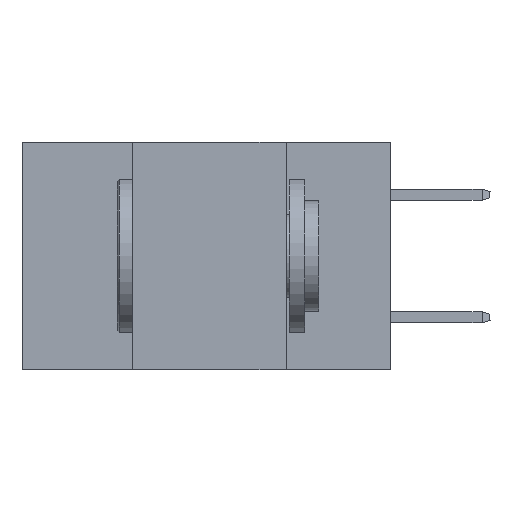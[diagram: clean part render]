
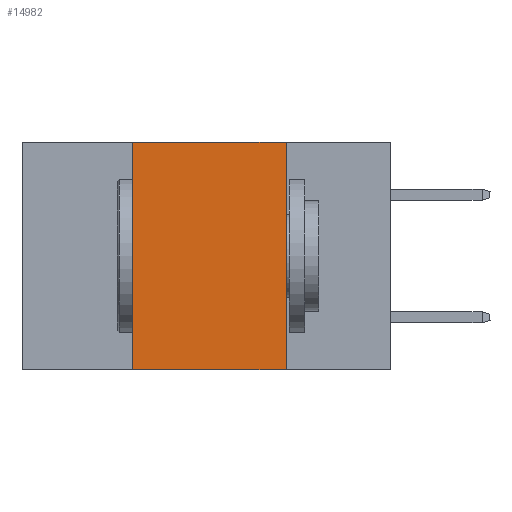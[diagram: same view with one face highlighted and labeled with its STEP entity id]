
A CAD part, left-side view. The second image highlights one B-rep face of the part: STEP entity #14982.
In plain terms, the highlighted planar face has unit normal (-1, 0, 0).
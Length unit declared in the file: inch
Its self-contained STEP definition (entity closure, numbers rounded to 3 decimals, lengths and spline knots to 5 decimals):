
#922 = LINE ( 'NONE', #15376, #20779 ) ;
#1189 = VERTEX_POINT ( 'NONE', #2346 ) ;
#2302 = VECTOR ( 'NONE', #21857, 39.37008 ) ;
#2346 = CARTESIAN_POINT ( 'NONE',  ( 0., 0.17, 0. ) ) ;
#4217 = ORIENTED_EDGE ( 'NONE', *, *, #22696, .T. ) ;
#4529 = EDGE_CURVE ( 'NONE', #16996, #1189, #922, .T. ) ;
#5674 = EDGE_LOOP ( 'NONE', ( #9450, #23091, #29783, #4217 ) ) ;
#6110 = VECTOR ( 'NONE', #13089, 39.37008 ) ;
#7836 = DIRECTION ( 'NONE',  ( 0., 0., -1. ) ) ;
#8096 = PLANE ( 'NONE',  #11311 ) ;
#9225 = LINE ( 'NONE', #26853, #2302 ) ;
#9450 = ORIENTED_EDGE ( 'NONE', *, *, #32554, .F. ) ;
#11311 = AXIS2_PLACEMENT_3D ( 'NONE', #15668, #30982, #15769 ) ;
#12926 = CARTESIAN_POINT ( 'NONE',  ( 0., 0.17, 0. ) ) ;
#13089 = DIRECTION ( 'NONE',  ( 0., -1., 0. ) ) ;
#14982 = ADVANCED_FACE ( 'NONE', ( #21894 ), #8096, .F. ) ;
#15376 = CARTESIAN_POINT ( 'NONE',  ( 0., 0.6, 0. ) ) ;
#15668 = CARTESIAN_POINT ( 'NONE',  ( 0., 0.6, 0. ) ) ;
#15769 = DIRECTION ( 'NONE',  ( 0., 0., -1. ) ) ;
#16996 = VERTEX_POINT ( 'NONE', #32463 ) ;
#20542 = DIRECTION ( 'NONE',  ( 0., -1., 0. ) ) ;
#20779 = VECTOR ( 'NONE', #20542, 39.37008 ) ;
#21857 = DIRECTION ( 'NONE',  ( 0., 0., 1. ) ) ;
#21894 = FACE_OUTER_BOUND ( 'NONE', #5674, .T. ) ;
#22696 = EDGE_CURVE ( 'NONE', #25229, #26412, #33141, .T. ) ;
#23091 = ORIENTED_EDGE ( 'NONE', *, *, #4529, .F. ) ;
#23609 = VECTOR ( 'NONE', #7836, 39.37008 ) ;
#25229 = VERTEX_POINT ( 'NONE', #28031 ) ;
#25867 = CARTESIAN_POINT ( 'NONE',  ( 0., 0.6, -0.37 ) ) ;
#26372 = CARTESIAN_POINT ( 'NONE',  ( 0., 0.17, -0.37 ) ) ;
#26412 = VERTEX_POINT ( 'NONE', #26372 ) ;
#26853 = CARTESIAN_POINT ( 'NONE',  ( 0., 0.42, 0. ) ) ;
#28031 = CARTESIAN_POINT ( 'NONE',  ( 0., 0.42, -0.37 ) ) ;
#29230 = EDGE_CURVE ( 'NONE', #25229, #16996, #9225, .T. ) ;
#29783 = ORIENTED_EDGE ( 'NONE', *, *, #29230, .F. ) ;
#30264 = LINE ( 'NONE', #12926, #23609 ) ;
#30982 = DIRECTION ( 'NONE',  ( 1., 0., 0. ) ) ;
#32463 = CARTESIAN_POINT ( 'NONE',  ( 0., 0.42, 0. ) ) ;
#32554 = EDGE_CURVE ( 'NONE', #1189, #26412, #30264, .T. ) ;
#33141 = LINE ( 'NONE', #25867, #6110 ) ;
